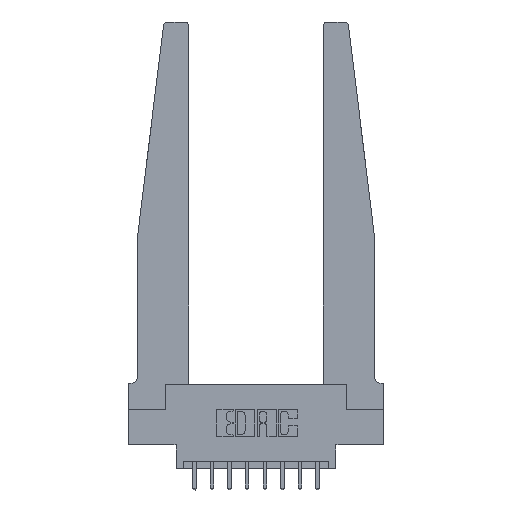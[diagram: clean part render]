
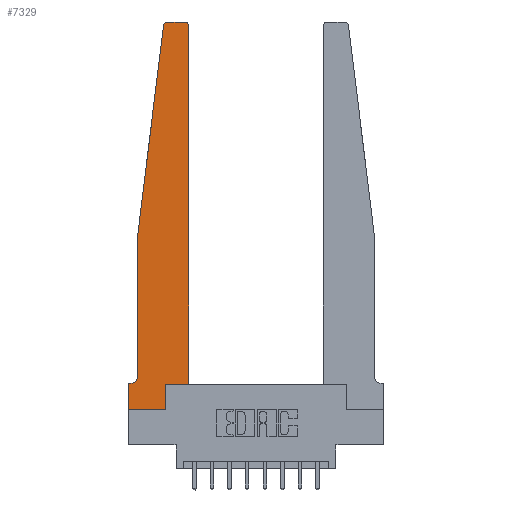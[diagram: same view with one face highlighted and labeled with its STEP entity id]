
A CAD part, top view. The second image highlights one B-rep face of the part: STEP entity #7329.
In plain terms, the highlighted planar face has unit normal (0, 0, 1).
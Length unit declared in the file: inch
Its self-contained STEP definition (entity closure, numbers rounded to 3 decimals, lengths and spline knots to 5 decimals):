
#237 = EDGE_CURVE ( 'NONE', #3791, #2174, #8162, .T. ) ;
#424 = VECTOR ( 'NONE', #3543, 39.37008 ) ;
#795 = LINE ( 'NONE', #4306, #6135 ) ;
#855 = CIRCLE ( 'NONE', #14704, 0.05 ) ;
#895 = DIRECTION ( 'NONE',  ( 0., 1., 0. ) ) ;
#919 = AXIS2_PLACEMENT_3D ( 'NONE', #13500, #6712, #14627 ) ;
#1357 = VECTOR ( 'NONE', #8579, 39.37008 ) ;
#1429 = EDGE_CURVE ( 'NONE', #6787, #8327, #6381, .T. ) ;
#1499 = ORIENTED_EDGE ( 'NONE', *, *, #237, .T. ) ;
#1573 = ORIENTED_EDGE ( 'NONE', *, *, #3066, .T. ) ;
#1623 = EDGE_CURVE ( 'NONE', #10031, #13056, #855, .T. ) ;
#1712 = LINE ( 'NONE', #13131, #1357 ) ;
#1783 = VECTOR ( 'NONE', #9920, 39.37008 ) ;
#1893 = DIRECTION ( 'NONE',  ( 0., 1., 0. ) ) ;
#2018 = AXIS2_PLACEMENT_3D ( 'NONE', #7933, #9062, #2290 ) ;
#2174 = VERTEX_POINT ( 'NONE', #2565 ) ;
#2193 = CARTESIAN_POINT ( 'NONE',  ( 0.395, 2.72, 0.37 ) ) ;
#2207 = CARTESIAN_POINT ( 'NONE',  ( 0.2605, 0.18, 0.37 ) ) ;
#2239 = PLANE ( 'NONE',  #2018 ) ;
#2290 = DIRECTION ( 'NONE',  ( 1., 0., 0. ) ) ;
#2383 = CARTESIAN_POINT ( 'NONE',  ( 0.015, 0.2375, 0.37 ) ) ;
#2492 = CARTESIAN_POINT ( 'NONE',  ( 0.2605, 0., 0.37 ) ) ;
#2565 = CARTESIAN_POINT ( 'NONE',  ( 0., 0., 0.37 ) ) ;
#2824 = EDGE_CURVE ( 'NONE', #13056, #3791, #1712, .T. ) ;
#2860 = CARTESIAN_POINT ( 'NONE',  ( 0.425, 0.18, 0.37 ) ) ;
#3066 = EDGE_CURVE ( 'NONE', #6605, #11092, #10581, .T. ) ;
#3328 = DIRECTION ( 'NONE',  ( 1., 0., 0. ) ) ;
#3347 = VECTOR ( 'NONE', #895, 39.37008 ) ;
#3375 = VECTOR ( 'NONE', #1893, 39.37008 ) ;
#3394 = CARTESIAN_POINT ( 'NONE',  ( 0., 0.1875, 0.37 ) ) ;
#3516 = DIRECTION ( 'NONE',  ( -1., 0., 0. ) ) ;
#3543 = DIRECTION ( 'NONE',  ( -1., 0., 0. ) ) ;
#3733 = LINE ( 'NONE', #8625, #3375 ) ;
#3791 = VERTEX_POINT ( 'NONE', #3394 ) ;
#3874 = EDGE_CURVE ( 'NONE', #11092, #5584, #9153, .T. ) ;
#4168 = AXIS2_PLACEMENT_3D ( 'NONE', #2193, #10131, #3328 ) ;
#4202 = EDGE_CURVE ( 'NONE', #11045, #11230, #8611, .T. ) ;
#4306 = CARTESIAN_POINT ( 'NONE',  ( 0.065, 1.25, 0.37 ) ) ;
#4338 = ORIENTED_EDGE ( 'NONE', *, *, #7721, .T. ) ;
#4969 = VECTOR ( 'NONE', #6355, 39.37008 ) ;
#5202 = CARTESIAN_POINT ( 'NONE',  ( 0., 0., 0.37 ) ) ;
#5248 = CARTESIAN_POINT ( 'NONE',  ( 0.395, 2.75, 0.37 ) ) ;
#5538 = CARTESIAN_POINT ( 'NONE',  ( 0.065, 1.25, 0.37 ) ) ;
#5539 = CIRCLE ( 'NONE', #919, 0.03 ) ;
#5584 = VERTEX_POINT ( 'NONE', #11509 ) ;
#5679 = LINE ( 'NONE', #5202, #4969 ) ;
#5802 = EDGE_LOOP ( 'NONE', ( #12793, #8269, #12685, #8559, #13417, #12871, #1499, #4338, #10585, #6313, #14050, #1573 ) ) ;
#6135 = VECTOR ( 'NONE', #11151, 39.37008 ) ;
#6313 = ORIENTED_EDGE ( 'NONE', *, *, #7075, .T. ) ;
#6334 = DIRECTION ( 'NONE',  ( -0.122, -0.992, 0. ) ) ;
#6355 = DIRECTION ( 'NONE',  ( 1., 0., 0. ) ) ;
#6381 = LINE ( 'NONE', #12231, #3347 ) ;
#6421 = VERTEX_POINT ( 'NONE', #2860 ) ;
#6605 = VERTEX_POINT ( 'NONE', #14606 ) ;
#6712 = DIRECTION ( 'NONE',  ( 0., 0., 1. ) ) ;
#6787 = VERTEX_POINT ( 'NONE', #2492 ) ;
#7075 = EDGE_CURVE ( 'NONE', #8327, #6421, #12452, .T. ) ;
#7082 = EDGE_CURVE ( 'NONE', #6421, #6605, #3733, .T. ) ;
#7329 = ADVANCED_FACE ( 'NONE', ( #9574 ), #2239, .T. ) ;
#7721 = EDGE_CURVE ( 'NONE', #2174, #6787, #5679, .T. ) ;
#7933 = CARTESIAN_POINT ( 'NONE',  ( 0., 0.1875, 0.37 ) ) ;
#8162 = LINE ( 'NONE', #10913, #1783 ) ;
#8269 = ORIENTED_EDGE ( 'NONE', *, *, #13421, .T. ) ;
#8327 = VERTEX_POINT ( 'NONE', #2207 ) ;
#8500 = CARTESIAN_POINT ( 'NONE',  ( 0.24675, 2.72367, 0.37 ) ) ;
#8559 = ORIENTED_EDGE ( 'NONE', *, *, #11185, .T. ) ;
#8579 = DIRECTION ( 'NONE',  ( -1., 0., 0. ) ) ;
#8611 = LINE ( 'NONE', #14245, #11299 ) ;
#8625 = CARTESIAN_POINT ( 'NONE',  ( 0.425, 0.18, 0.37 ) ) ;
#9062 = DIRECTION ( 'NONE',  ( 0., 0., 1. ) ) ;
#9153 = LINE ( 'NONE', #10344, #424 ) ;
#9321 = CARTESIAN_POINT ( 'NONE',  ( 0.015, 0.1875, 0.37 ) ) ;
#9411 = VECTOR ( 'NONE', #14339, 39.37008 ) ;
#9574 = FACE_OUTER_BOUND ( 'NONE', #5802, .T. ) ;
#9782 = CARTESIAN_POINT ( 'NONE',  ( 0.425, 0.18, 0.37 ) ) ;
#9920 = DIRECTION ( 'NONE',  ( 0., -1., 0. ) ) ;
#10031 = VERTEX_POINT ( 'NONE', #13320 ) ;
#10131 = DIRECTION ( 'NONE',  ( 0., 0., 1. ) ) ;
#10322 = DIRECTION ( 'NONE',  ( 0., 0., -1. ) ) ;
#10344 = CARTESIAN_POINT ( 'NONE',  ( 0.25, 2.75, 0.37 ) ) ;
#10581 = CIRCLE ( 'NONE', #4168, 0.03 ) ;
#10585 = ORIENTED_EDGE ( 'NONE', *, *, #1429, .T. ) ;
#10913 = CARTESIAN_POINT ( 'NONE',  ( 0., 0., 0.37 ) ) ;
#11045 = VERTEX_POINT ( 'NONE', #8500 ) ;
#11092 = VERTEX_POINT ( 'NONE', #5248 ) ;
#11151 = DIRECTION ( 'NONE',  ( 0., -1., 0. ) ) ;
#11185 = EDGE_CURVE ( 'NONE', #11230, #10031, #795, .T. ) ;
#11230 = VERTEX_POINT ( 'NONE', #5538 ) ;
#11299 = VECTOR ( 'NONE', #6334, 39.37008 ) ;
#11509 = CARTESIAN_POINT ( 'NONE',  ( 0.27653, 2.75, 0.37 ) ) ;
#12231 = CARTESIAN_POINT ( 'NONE',  ( 0.2605, 0.18, 0.37 ) ) ;
#12452 = LINE ( 'NONE', #9782, #9411 ) ;
#12685 = ORIENTED_EDGE ( 'NONE', *, *, #4202, .T. ) ;
#12793 = ORIENTED_EDGE ( 'NONE', *, *, #3874, .T. ) ;
#12871 = ORIENTED_EDGE ( 'NONE', *, *, #2824, .T. ) ;
#13056 = VERTEX_POINT ( 'NONE', #9321 ) ;
#13131 = CARTESIAN_POINT ( 'NONE',  ( 0.065, 0.1875, 0.37 ) ) ;
#13320 = CARTESIAN_POINT ( 'NONE',  ( 0.065, 0.2375, 0.37 ) ) ;
#13417 = ORIENTED_EDGE ( 'NONE', *, *, #1623, .T. ) ;
#13421 = EDGE_CURVE ( 'NONE', #5584, #11045, #5539, .T. ) ;
#13500 = CARTESIAN_POINT ( 'NONE',  ( 0.27653, 2.72, 0.37 ) ) ;
#14050 = ORIENTED_EDGE ( 'NONE', *, *, #7082, .T. ) ;
#14245 = CARTESIAN_POINT ( 'NONE',  ( 0.065, 1.25, 0.37 ) ) ;
#14339 = DIRECTION ( 'NONE',  ( 1., 0., 0. ) ) ;
#14606 = CARTESIAN_POINT ( 'NONE',  ( 0.425, 2.72, 0.37 ) ) ;
#14627 = DIRECTION ( 'NONE',  ( 1., 0., 0. ) ) ;
#14704 = AXIS2_PLACEMENT_3D ( 'NONE', #2383, #10322, #3516 ) ;
